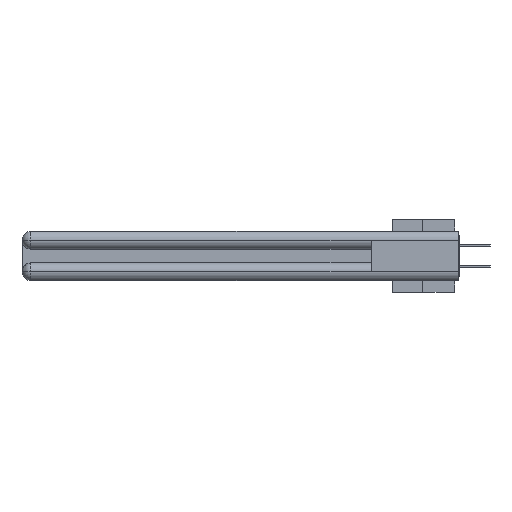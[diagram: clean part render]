
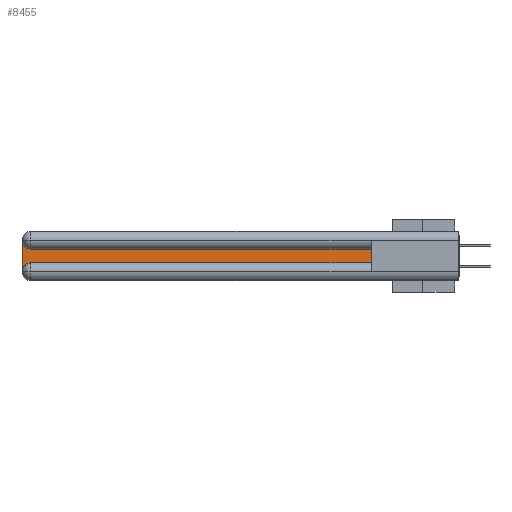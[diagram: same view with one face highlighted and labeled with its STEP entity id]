
A CAD part, left-side view. The second image highlights one B-rep face of the part: STEP entity #8455.
In plain terms, the highlighted planar face has unit normal (-1, 0, 0).
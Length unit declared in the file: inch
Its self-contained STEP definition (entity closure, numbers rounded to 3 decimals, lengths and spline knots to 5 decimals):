
#344 = VERTEX_POINT ( 'NONE', #24713 ) ;
#1232 = VERTEX_POINT ( 'NONE', #6404 ) ;
#1336 = LINE ( 'NONE', #7141, #17649 ) ;
#1789 = CARTESIAN_POINT ( 'NONE',  ( 0.075, 2.94, -0.2775 ) ) ;
#1827 = EDGE_LOOP ( 'NONE', ( #31667, #33874, #5121, #32466, #7496, #35173 ) ) ;
#5121 = ORIENTED_EDGE ( 'NONE', *, *, #9146, .T. ) ;
#5496 = EDGE_CURVE ( 'NONE', #33867, #6378, #20826, .T. ) ;
#6378 = VERTEX_POINT ( 'NONE', #11076 ) ;
#6404 = CARTESIAN_POINT ( 'NONE',  ( 0.075, 0.6, -0.2175 ) ) ;
#7141 = CARTESIAN_POINT ( 'NONE',  ( 0.075, 0.6, -0.1225 ) ) ;
#7496 = ORIENTED_EDGE ( 'NONE', *, *, #28628, .T. ) ;
#7724 = CARTESIAN_POINT ( 'NONE',  ( 0.075, 0.6, -0.1225 ) ) ;
#8431 = CARTESIAN_POINT ( 'NONE',  ( 0.075, 3., -0.2775 ) ) ;
#8455 = ADVANCED_FACE ( 'NONE', ( #31189 ), #30984, .F. ) ;
#9146 = EDGE_CURVE ( 'NONE', #30875, #33867, #20865, .T. ) ;
#9446 = DIRECTION ( 'NONE',  ( 1., 0., 0. ) ) ;
#11076 = CARTESIAN_POINT ( 'NONE',  ( 0.075, 2.94, -0.2175 ) ) ;
#12383 = CARTESIAN_POINT ( 'NONE',  ( 0.075, 0.6, -0.2175 ) ) ;
#14181 = CARTESIAN_POINT ( 'NONE',  ( 0.075, 3., -0.0625 ) ) ;
#14896 = DIRECTION ( 'NONE',  ( 0., 1., 0. ) ) ;
#16566 = VECTOR ( 'NONE', #23894, 39.37008 ) ;
#17649 = VECTOR ( 'NONE', #14896, 39.37008 ) ;
#17828 = DIRECTION ( 'NONE',  ( 1., 0., 0. ) ) ;
#17903 = CARTESIAN_POINT ( 'NONE',  ( 0.075, 2.94, -0.0625 ) ) ;
#18113 = LINE ( 'NONE', #31873, #29711 ) ;
#18525 = VECTOR ( 'NONE', #31397, 39.37008 ) ;
#19719 = AXIS2_PLACEMENT_3D ( 'NONE', #25860, #9446, #25751 ) ;
#19881 = AXIS2_PLACEMENT_3D ( 'NONE', #1789, #17828, #31585 ) ;
#20826 = CIRCLE ( 'NONE', #19881, 0.06 ) ;
#20865 = LINE ( 'NONE', #23414, #16566 ) ;
#23267 = LINE ( 'NONE', #12383, #18525 ) ;
#23414 = CARTESIAN_POINT ( 'NONE',  ( 0.075, 3., -0.2175 ) ) ;
#23894 = DIRECTION ( 'NONE',  ( 0., 0., -1. ) ) ;
#24026 = DIRECTION ( 'NONE',  ( 0., 0., 1. ) ) ;
#24483 = VERTEX_POINT ( 'NONE', #7724 ) ;
#24713 = CARTESIAN_POINT ( 'NONE',  ( 0.075, 2.94, -0.1225 ) ) ;
#25751 = DIRECTION ( 'NONE',  ( 0., 0., -1. ) ) ;
#25860 = CARTESIAN_POINT ( 'NONE',  ( 0.075, 3., -0.1225 ) ) ;
#26086 = DIRECTION ( 'NONE',  ( 0., 0., -1. ) ) ;
#28628 = EDGE_CURVE ( 'NONE', #6378, #1232, #23267, .T. ) ;
#28710 = EDGE_CURVE ( 'NONE', #24483, #344, #1336, .T. ) ;
#29711 = VECTOR ( 'NONE', #24026, 39.37008 ) ;
#30875 = VERTEX_POINT ( 'NONE', #14181 ) ;
#30984 = PLANE ( 'NONE',  #19719 ) ;
#31189 = FACE_OUTER_BOUND ( 'NONE', #1827, .T. ) ;
#31195 = DIRECTION ( 'NONE',  ( 1., 0., 0. ) ) ;
#31397 = DIRECTION ( 'NONE',  ( 0., -1., 0. ) ) ;
#31585 = DIRECTION ( 'NONE',  ( 0., 0., -1. ) ) ;
#31667 = ORIENTED_EDGE ( 'NONE', *, *, #28710, .T. ) ;
#31873 = CARTESIAN_POINT ( 'NONE',  ( 0.075, 0.6, -0.2175 ) ) ;
#32466 = ORIENTED_EDGE ( 'NONE', *, *, #5496, .T. ) ;
#32811 = AXIS2_PLACEMENT_3D ( 'NONE', #17903, #31195, #26086 ) ;
#32866 = EDGE_CURVE ( 'NONE', #344, #30875, #34016, .T. ) ;
#33639 = EDGE_CURVE ( 'NONE', #1232, #24483, #18113, .T. ) ;
#33867 = VERTEX_POINT ( 'NONE', #8431 ) ;
#33874 = ORIENTED_EDGE ( 'NONE', *, *, #32866, .T. ) ;
#34016 = CIRCLE ( 'NONE', #32811, 0.06 ) ;
#35173 = ORIENTED_EDGE ( 'NONE', *, *, #33639, .T. ) ;
